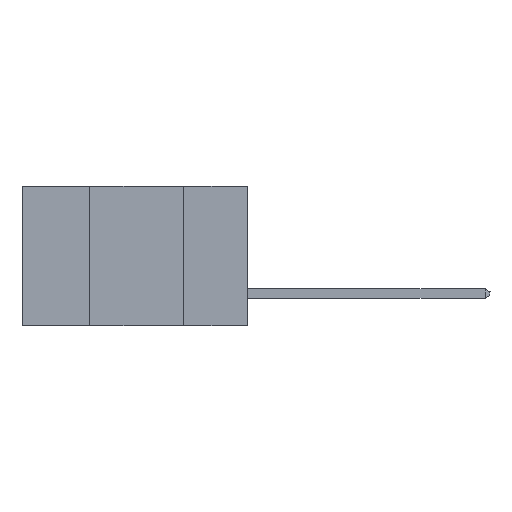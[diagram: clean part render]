
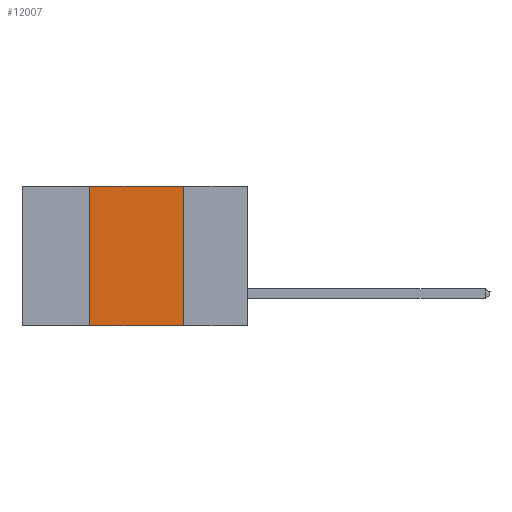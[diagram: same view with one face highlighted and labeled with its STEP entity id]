
A CAD part, left-side view. The second image highlights one B-rep face of the part: STEP entity #12007.
In plain terms, the highlighted planar face has unit normal (-1, 0, 0).
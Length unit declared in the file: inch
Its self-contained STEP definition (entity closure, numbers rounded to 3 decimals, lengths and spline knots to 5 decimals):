
#69 = CARTESIAN_POINT ( 'NONE',  ( 0., 0.6, -0.37 ) ) ;
#238 = CARTESIAN_POINT ( 'NONE',  ( 0., 0.17, 0. ) ) ;
#1288 = DIRECTION ( 'NONE',  ( 0., -1., 0. ) ) ;
#1383 = CARTESIAN_POINT ( 'NONE',  ( 0., 0.42, -0.37 ) ) ;
#2163 = AXIS2_PLACEMENT_3D ( 'NONE', #6585, #5444, #5684 ) ;
#2516 = VECTOR ( 'NONE', #10171, 39.37008 ) ;
#2966 = DIRECTION ( 'NONE',  ( 0., 0., -1. ) ) ;
#3149 = VECTOR ( 'NONE', #2966, 39.37008 ) ;
#3625 = LINE ( 'NONE', #69, #12762 ) ;
#3803 = VECTOR ( 'NONE', #1288, 39.37008 ) ;
#3936 = EDGE_LOOP ( 'NONE', ( #9105, #15204, #9480, #11018 ) ) ;
#4177 = LINE ( 'NONE', #8919, #3803 ) ;
#4216 = FACE_OUTER_BOUND ( 'NONE', #3936, .T. ) ;
#5279 = LINE ( 'NONE', #6504, #3149 ) ;
#5444 = DIRECTION ( 'NONE',  ( 1., 0., 0. ) ) ;
#5684 = DIRECTION ( 'NONE',  ( 0., 0., -1. ) ) ;
#5765 = EDGE_CURVE ( 'NONE', #9106, #10562, #3625, .T. ) ;
#6504 = CARTESIAN_POINT ( 'NONE',  ( 0., 0.17, -0.37 ) ) ;
#6585 = CARTESIAN_POINT ( 'NONE',  ( 0., 0.6, 0. ) ) ;
#8542 = EDGE_CURVE ( 'NONE', #10217, #10562, #5279, .T. ) ;
#8694 = DIRECTION ( 'NONE',  ( 0., -1., 0. ) ) ;
#8919 = CARTESIAN_POINT ( 'NONE',  ( 0., 0.6, 0. ) ) ;
#8945 = VERTEX_POINT ( 'NONE', #15070 ) ;
#9105 = ORIENTED_EDGE ( 'NONE', *, *, #8542, .F. ) ;
#9106 = VERTEX_POINT ( 'NONE', #10484 ) ;
#9480 = ORIENTED_EDGE ( 'NONE', *, *, #14906, .F. ) ;
#9658 = CARTESIAN_POINT ( 'NONE',  ( 0., 0.17, -0.37 ) ) ;
#10171 = DIRECTION ( 'NONE',  ( 0., 0., 1. ) ) ;
#10217 = VERTEX_POINT ( 'NONE', #238 ) ;
#10484 = CARTESIAN_POINT ( 'NONE',  ( 0., 0.42, -0.37 ) ) ;
#10562 = VERTEX_POINT ( 'NONE', #9658 ) ;
#10743 = EDGE_CURVE ( 'NONE', #8945, #10217, #4177, .T. ) ;
#11018 = ORIENTED_EDGE ( 'NONE', *, *, #5765, .T. ) ;
#11659 = PLANE ( 'NONE',  #2163 ) ;
#12007 = ADVANCED_FACE ( 'NONE', ( #4216 ), #11659, .F. ) ;
#12762 = VECTOR ( 'NONE', #8694, 39.37008 ) ;
#14906 = EDGE_CURVE ( 'NONE', #9106, #8945, #14923, .T. ) ;
#14923 = LINE ( 'NONE', #1383, #2516 ) ;
#15070 = CARTESIAN_POINT ( 'NONE',  ( 0., 0.42, 0. ) ) ;
#15204 = ORIENTED_EDGE ( 'NONE', *, *, #10743, .F. ) ;
